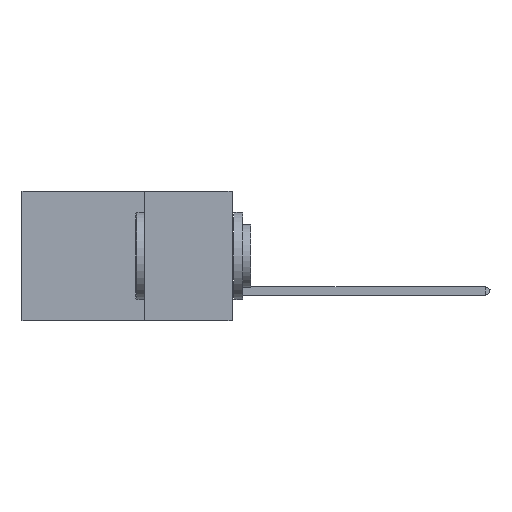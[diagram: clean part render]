
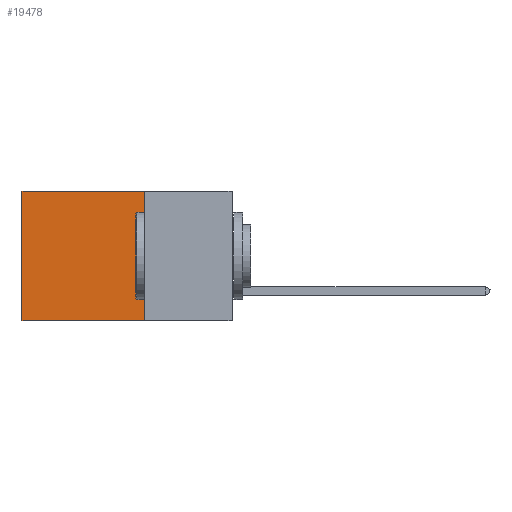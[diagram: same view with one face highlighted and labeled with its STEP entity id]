
A CAD part, left-side view. The second image highlights one B-rep face of the part: STEP entity #19478.
In plain terms, the highlighted planar face has unit normal (-1, 0, 0).
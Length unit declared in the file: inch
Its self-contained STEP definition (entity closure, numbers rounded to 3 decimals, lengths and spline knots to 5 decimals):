
#728 = CARTESIAN_POINT ( 'NONE',  ( 0.2875, 0.6, -0.37 ) ) ;
#1476 = VECTOR ( 'NONE', #18354, 39.37008 ) ;
#1731 = ORIENTED_EDGE ( 'NONE', *, *, #6170, .F. ) ;
#2053 = EDGE_CURVE ( 'NONE', #4812, #5537, #19026, .T. ) ;
#3404 = DIRECTION ( 'NONE',  ( 0., 1., 0. ) ) ;
#3838 = PLANE ( 'NONE',  #28116 ) ;
#4240 = CARTESIAN_POINT ( 'NONE',  ( 0.2875, 0.25, 0. ) ) ;
#4812 = VERTEX_POINT ( 'NONE', #31834 ) ;
#5537 = VERTEX_POINT ( 'NONE', #15465 ) ;
#6170 = EDGE_CURVE ( 'NONE', #5537, #6665, #9972, .T. ) ;
#6614 = EDGE_CURVE ( 'NONE', #25374, #6665, #12297, .T. ) ;
#6665 = VERTEX_POINT ( 'NONE', #728 ) ;
#9972 = LINE ( 'NONE', #21653, #38648 ) ;
#10788 = VECTOR ( 'NONE', #21973, 39.37008 ) ;
#11976 = VECTOR ( 'NONE', #12446, 39.37008 ) ;
#12297 = LINE ( 'NONE', #18745, #1476 ) ;
#12446 = DIRECTION ( 'NONE',  ( 0., 0., -1. ) ) ;
#12897 = DIRECTION ( 'NONE',  ( 0., 0., -1. ) ) ;
#13504 = EDGE_CURVE ( 'NONE', #4812, #25374, #34274, .T. ) ;
#14320 = EDGE_LOOP ( 'NONE', ( #35909, #1731, #34648, #23705 ) ) ;
#15465 = CARTESIAN_POINT ( 'NONE',  ( 0.2875, 0.25, -0.37 ) ) ;
#15815 = CARTESIAN_POINT ( 'NONE',  ( 0.2875, 0.25, 0. ) ) ;
#18354 = DIRECTION ( 'NONE',  ( 0., 0., -1. ) ) ;
#18745 = CARTESIAN_POINT ( 'NONE',  ( 0.2875, 0.6, 0. ) ) ;
#19026 = LINE ( 'NONE', #36609, #11976 ) ;
#19370 = DIRECTION ( 'NONE',  ( 1., 0., 0. ) ) ;
#19478 = ADVANCED_FACE ( 'NONE', ( #38412 ), #3838, .F. ) ;
#21653 = CARTESIAN_POINT ( 'NONE',  ( 0.2875, 0.25, -0.37 ) ) ;
#21973 = DIRECTION ( 'NONE',  ( 0., 1., 0. ) ) ;
#23705 = ORIENTED_EDGE ( 'NONE', *, *, #13504, .T. ) ;
#25064 = CARTESIAN_POINT ( 'NONE',  ( 0.2875, 0.6, 0. ) ) ;
#25374 = VERTEX_POINT ( 'NONE', #25064 ) ;
#28116 = AXIS2_PLACEMENT_3D ( 'NONE', #4240, #19370, #12897 ) ;
#31834 = CARTESIAN_POINT ( 'NONE',  ( 0.2875, 0.25, 0. ) ) ;
#34274 = LINE ( 'NONE', #15815, #10788 ) ;
#34648 = ORIENTED_EDGE ( 'NONE', *, *, #2053, .F. ) ;
#35909 = ORIENTED_EDGE ( 'NONE', *, *, #6614, .T. ) ;
#36609 = CARTESIAN_POINT ( 'NONE',  ( 0.2875, 0.25, 0. ) ) ;
#38412 = FACE_OUTER_BOUND ( 'NONE', #14320, .T. ) ;
#38648 = VECTOR ( 'NONE', #3404, 39.37008 ) ;
